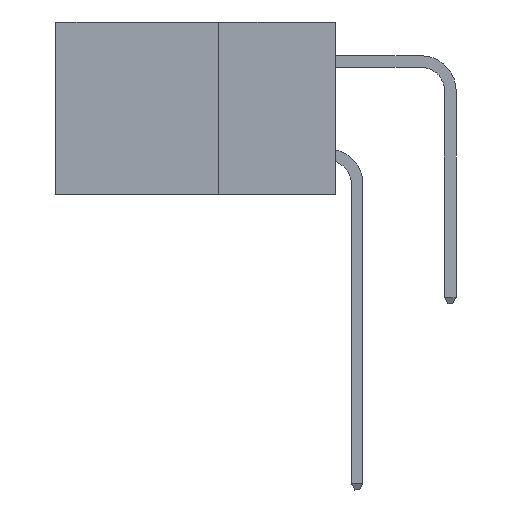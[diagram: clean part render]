
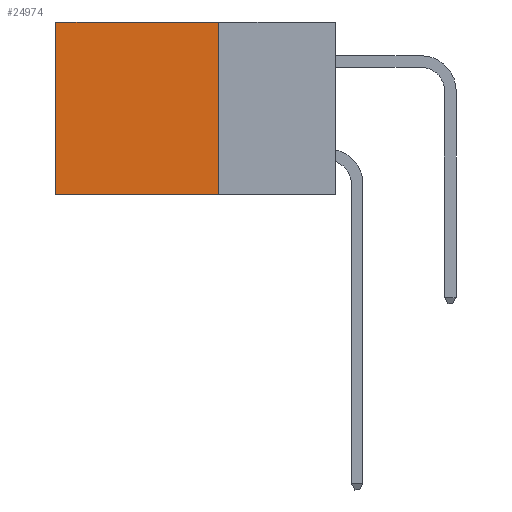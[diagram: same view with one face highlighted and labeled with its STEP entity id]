
A CAD part, left-side view. The second image highlights one B-rep face of the part: STEP entity #24974.
In plain terms, the highlighted planar face has unit normal (-1, 0, 0).
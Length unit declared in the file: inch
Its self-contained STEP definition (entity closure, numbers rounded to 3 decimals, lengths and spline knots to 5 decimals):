
#253 = VERTEX_POINT ( 'NONE', #15255 ) ;
#2203 = VERTEX_POINT ( 'NONE', #7777 ) ;
#2435 = ORIENTED_EDGE ( 'NONE', *, *, #3398, .F. ) ;
#3398 = EDGE_CURVE ( 'NONE', #2203, #253, #20637, .T. ) ;
#3637 = CARTESIAN_POINT ( 'NONE',  ( 0.2875, 0.25, 0. ) ) ;
#4181 = CARTESIAN_POINT ( 'NONE',  ( 0.2875, 0.6, -0.37 ) ) ;
#4460 = DIRECTION ( 'NONE',  ( 0., 0., -1. ) ) ;
#5045 = ORIENTED_EDGE ( 'NONE', *, *, #21474, .T. ) ;
#5562 = LINE ( 'NONE', #16809, #12632 ) ;
#5784 = AXIS2_PLACEMENT_3D ( 'NONE', #3637, #11372, #7424 ) ;
#6877 = DIRECTION ( 'NONE',  ( 0., 1., 0. ) ) ;
#7424 = DIRECTION ( 'NONE',  ( 0., 0., -1. ) ) ;
#7777 = CARTESIAN_POINT ( 'NONE',  ( 0.2875, 0.25, 0. ) ) ;
#9397 = LINE ( 'NONE', #16187, #17461 ) ;
#10077 = VECTOR ( 'NONE', #16830, 39.37008 ) ;
#10511 = FACE_OUTER_BOUND ( 'NONE', #18087, .T. ) ;
#11372 = DIRECTION ( 'NONE',  ( 1., 0., 0. ) ) ;
#12215 = VECTOR ( 'NONE', #4460, 39.37008 ) ;
#12314 = EDGE_CURVE ( 'NONE', #253, #20554, #15359, .T. ) ;
#12632 = VECTOR ( 'NONE', #6877, 39.37008 ) ;
#14569 = ORIENTED_EDGE ( 'NONE', *, *, #18741, .T. ) ;
#14753 = CARTESIAN_POINT ( 'NONE',  ( 0.2875, 0.25, -0.37 ) ) ;
#14831 = ORIENTED_EDGE ( 'NONE', *, *, #12314, .F. ) ;
#15255 = CARTESIAN_POINT ( 'NONE',  ( 0.2875, 0.25, -0.37 ) ) ;
#15359 = LINE ( 'NONE', #14753, #10077 ) ;
#15371 = PLANE ( 'NONE',  #5784 ) ;
#16187 = CARTESIAN_POINT ( 'NONE',  ( 0.2875, 0.6, 0. ) ) ;
#16256 = CARTESIAN_POINT ( 'NONE',  ( 0.2875, 0.6, 0. ) ) ;
#16292 = CARTESIAN_POINT ( 'NONE',  ( 0.2875, 0.25, 0. ) ) ;
#16809 = CARTESIAN_POINT ( 'NONE',  ( 0.2875, 0.25, 0. ) ) ;
#16830 = DIRECTION ( 'NONE',  ( 0., 1., 0. ) ) ;
#17461 = VECTOR ( 'NONE', #18435, 39.37008 ) ;
#18087 = EDGE_LOOP ( 'NONE', ( #5045, #14831, #2435, #14569 ) ) ;
#18435 = DIRECTION ( 'NONE',  ( 0., 0., -1. ) ) ;
#18741 = EDGE_CURVE ( 'NONE', #2203, #18937, #5562, .T. ) ;
#18937 = VERTEX_POINT ( 'NONE', #16256 ) ;
#20554 = VERTEX_POINT ( 'NONE', #4181 ) ;
#20637 = LINE ( 'NONE', #16292, #12215 ) ;
#21474 = EDGE_CURVE ( 'NONE', #18937, #20554, #9397, .T. ) ;
#24974 = ADVANCED_FACE ( 'NONE', ( #10511 ), #15371, .F. ) ;
